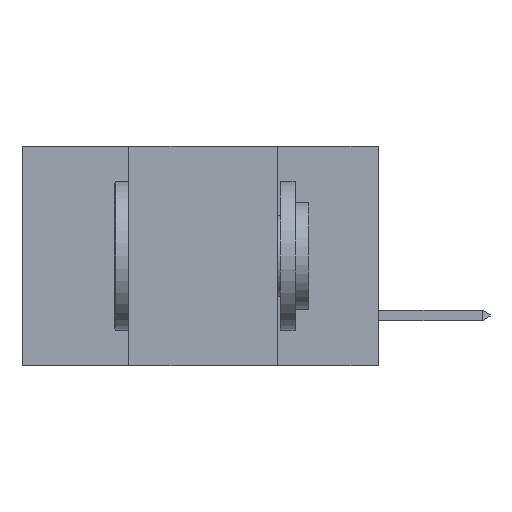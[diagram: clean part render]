
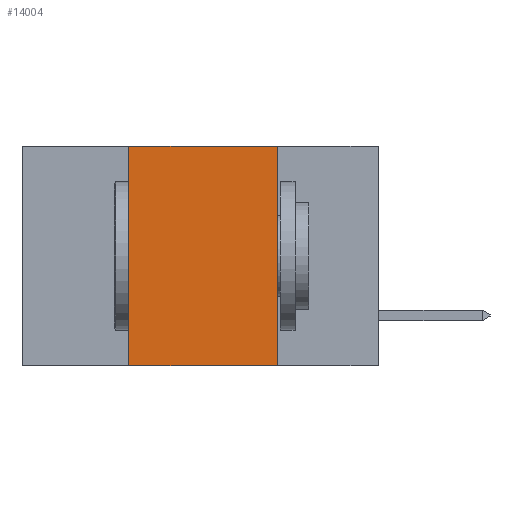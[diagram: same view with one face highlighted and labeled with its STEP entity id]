
A CAD part, left-side view. The second image highlights one B-rep face of the part: STEP entity #14004.
In plain terms, the highlighted planar face has unit normal (-1, 0, 0).
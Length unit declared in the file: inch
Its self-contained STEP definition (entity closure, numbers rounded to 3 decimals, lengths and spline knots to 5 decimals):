
#40 = EDGE_CURVE ( 'NONE', #20290, #13300, #19446, .T. ) ;
#673 = EDGE_LOOP ( 'NONE', ( #6197, #18579, #3995, #5528 ) ) ;
#1191 = CARTESIAN_POINT ( 'NONE',  ( 0., 0.6, 0. ) ) ;
#1360 = FACE_OUTER_BOUND ( 'NONE', #673, .T. ) ;
#1698 = CARTESIAN_POINT ( 'NONE',  ( 0., 0.17, -0.37 ) ) ;
#2488 = CARTESIAN_POINT ( 'NONE',  ( 0., 0.42, 0. ) ) ;
#2605 = VECTOR ( 'NONE', #14771, 39.37008 ) ;
#3335 = EDGE_CURVE ( 'NONE', #21011, #8619, #5874, .T. ) ;
#3578 = AXIS2_PLACEMENT_3D ( 'NONE', #9174, #20392, #10840 ) ;
#3995 = ORIENTED_EDGE ( 'NONE', *, *, #40, .F. ) ;
#5528 = ORIENTED_EDGE ( 'NONE', *, *, #16928, .T. ) ;
#5874 = LINE ( 'NONE', #11654, #17813 ) ;
#6197 = ORIENTED_EDGE ( 'NONE', *, *, #3335, .F. ) ;
#6504 = CARTESIAN_POINT ( 'NONE',  ( 0., 0.42, -0.37 ) ) ;
#6775 = LINE ( 'NONE', #1191, #10648 ) ;
#8391 = DIRECTION ( 'NONE',  ( 0., -1., 0. ) ) ;
#8619 = VERTEX_POINT ( 'NONE', #1698 ) ;
#9174 = CARTESIAN_POINT ( 'NONE',  ( 0., 0.6, 0. ) ) ;
#9960 = CARTESIAN_POINT ( 'NONE',  ( 0., 0.17, 0. ) ) ;
#10648 = VECTOR ( 'NONE', #19209, 39.37008 ) ;
#10840 = DIRECTION ( 'NONE',  ( 0., 0., -1. ) ) ;
#11254 = LINE ( 'NONE', #14822, #19275 ) ;
#11654 = CARTESIAN_POINT ( 'NONE',  ( 0., 0.17, 0. ) ) ;
#12876 = DIRECTION ( 'NONE',  ( 0., 0., -1. ) ) ;
#13300 = VERTEX_POINT ( 'NONE', #2488 ) ;
#14004 = ADVANCED_FACE ( 'NONE', ( #1360 ), #17218, .F. ) ;
#14771 = DIRECTION ( 'NONE',  ( 0., 0., 1. ) ) ;
#14822 = CARTESIAN_POINT ( 'NONE',  ( 0., 0.6, -0.37 ) ) ;
#15951 = CARTESIAN_POINT ( 'NONE',  ( 0., 0.42, 0. ) ) ;
#16928 = EDGE_CURVE ( 'NONE', #20290, #8619, #11254, .T. ) ;
#17218 = PLANE ( 'NONE',  #3578 ) ;
#17813 = VECTOR ( 'NONE', #12876, 39.37008 ) ;
#18579 = ORIENTED_EDGE ( 'NONE', *, *, #19203, .F. ) ;
#19203 = EDGE_CURVE ( 'NONE', #13300, #21011, #6775, .T. ) ;
#19209 = DIRECTION ( 'NONE',  ( 0., -1., 0. ) ) ;
#19275 = VECTOR ( 'NONE', #8391, 39.37008 ) ;
#19446 = LINE ( 'NONE', #15951, #2605 ) ;
#20290 = VERTEX_POINT ( 'NONE', #6504 ) ;
#20392 = DIRECTION ( 'NONE',  ( 1., 0., 0. ) ) ;
#21011 = VERTEX_POINT ( 'NONE', #9960 ) ;
